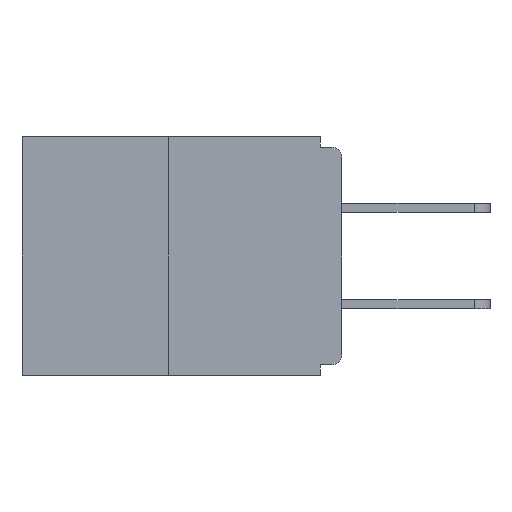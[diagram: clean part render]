
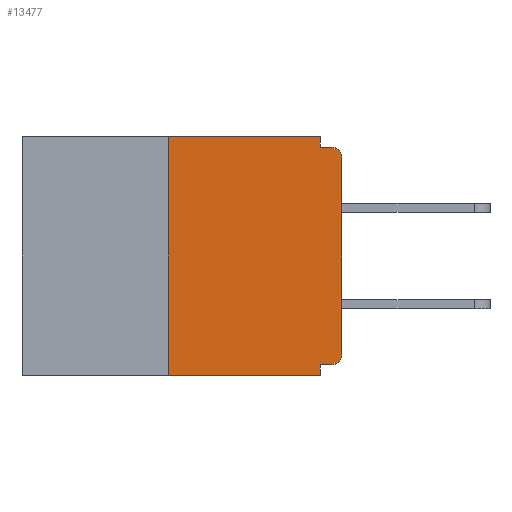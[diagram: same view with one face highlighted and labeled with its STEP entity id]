
A CAD part, left-side view. The second image highlights one B-rep face of the part: STEP entity #13477.
In plain terms, the highlighted planar face has unit normal (-1, 0, 0).
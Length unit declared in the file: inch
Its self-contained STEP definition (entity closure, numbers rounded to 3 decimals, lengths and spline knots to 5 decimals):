
#249 = CARTESIAN_POINT ( 'NONE',  ( 0., 0., -0.328 ) ) ;
#279 = DIRECTION ( 'NONE',  ( -1., 0., 0. ) ) ;
#351 = VERTEX_POINT ( 'NONE', #12477 ) ;
#446 = EDGE_CURVE ( 'NONE', #6713, #351, #14507, .T. ) ;
#727 = CARTESIAN_POINT ( 'NONE',  ( 0., 0.25, 0. ) ) ;
#910 = EDGE_CURVE ( 'NONE', #2890, #11654, #1604, .T. ) ;
#1026 = CARTESIAN_POINT ( 'NONE',  ( 0., 0.015, -0.015 ) ) ;
#1099 = ORIENTED_EDGE ( 'NONE', *, *, #910, .T. ) ;
#1271 = VERTEX_POINT ( 'NONE', #4079 ) ;
#1514 = DIRECTION ( 'NONE',  ( 0., 0., -1. ) ) ;
#1546 = AXIS2_PLACEMENT_3D ( 'NONE', #13833, #2771, #2620 ) ;
#1586 = CARTESIAN_POINT ( 'NONE',  ( 0., 0.031, -0.343 ) ) ;
#1604 = LINE ( 'NONE', #2665, #3016 ) ;
#1802 = DIRECTION ( 'NONE',  ( 0., 0., -1. ) ) ;
#1822 = DIRECTION ( 'NONE',  ( 0., 0., 1. ) ) ;
#2344 = VERTEX_POINT ( 'NONE', #13068 ) ;
#2375 = FACE_OUTER_BOUND ( 'NONE', #13878, .T. ) ;
#2427 = CIRCLE ( 'NONE', #1546, 0.015 ) ;
#2615 = DIRECTION ( 'NONE',  ( 0., -1., 0. ) ) ;
#2620 = DIRECTION ( 'NONE',  ( 0., 0., -1. ) ) ;
#2665 = CARTESIAN_POINT ( 'NONE',  ( 0., 0.46, -0.343 ) ) ;
#2771 = DIRECTION ( 'NONE',  ( -1., 0., 0. ) ) ;
#2811 = DIRECTION ( 'NONE',  ( 1., 0., 0. ) ) ;
#2890 = VERTEX_POINT ( 'NONE', #10307 ) ;
#2918 = VECTOR ( 'NONE', #1514, 39.37008 ) ;
#2968 = LINE ( 'NONE', #11982, #5103 ) ;
#3007 = AXIS2_PLACEMENT_3D ( 'NONE', #3463, #279, #7038 ) ;
#3016 = VECTOR ( 'NONE', #2615, 39.37008 ) ;
#3120 = LINE ( 'NONE', #3631, #12502 ) ;
#3336 = ORIENTED_EDGE ( 'NONE', *, *, #10011, .F. ) ;
#3463 = CARTESIAN_POINT ( 'NONE',  ( 0., 0.015, -0.03 ) ) ;
#3493 = EDGE_CURVE ( 'NONE', #2344, #8416, #2968, .T. ) ;
#3596 = CARTESIAN_POINT ( 'NONE',  ( 0., 0.031, -0.343 ) ) ;
#3631 = CARTESIAN_POINT ( 'NONE',  ( 0., 0.031, 0. ) ) ;
#4079 = CARTESIAN_POINT ( 'NONE',  ( 0., 0., -0.03 ) ) ;
#4272 = LINE ( 'NONE', #10530, #12057 ) ;
#4614 = DIRECTION ( 'NONE',  ( 0., 0., -1. ) ) ;
#4646 = VECTOR ( 'NONE', #7058, 39.37008 ) ;
#5100 = VERTEX_POINT ( 'NONE', #10645 ) ;
#5103 = VECTOR ( 'NONE', #10808, 39.37008 ) ;
#5326 = CARTESIAN_POINT ( 'NONE',  ( 0., 0.031, -0.015 ) ) ;
#5466 = AXIS2_PLACEMENT_3D ( 'NONE', #6154, #2811, #1802 ) ;
#5928 = ORIENTED_EDGE ( 'NONE', *, *, #12343, .F. ) ;
#5972 = EDGE_CURVE ( 'NONE', #1271, #14247, #12173, .T. ) ;
#6154 = CARTESIAN_POINT ( 'NONE',  ( 0., 0.46, 0. ) ) ;
#6713 = VERTEX_POINT ( 'NONE', #9523 ) ;
#6881 = DIRECTION ( 'NONE',  ( 0., 0., 1. ) ) ;
#6967 = ORIENTED_EDGE ( 'NONE', *, *, #11151, .T. ) ;
#7038 = DIRECTION ( 'NONE',  ( 0., 0., -1. ) ) ;
#7058 = DIRECTION ( 'NONE',  ( 0., 1., 0. ) ) ;
#8039 = ORIENTED_EDGE ( 'NONE', *, *, #5972, .T. ) ;
#8416 = VERTEX_POINT ( 'NONE', #11031 ) ;
#9334 = VECTOR ( 'NONE', #1822, 39.37008 ) ;
#9523 = CARTESIAN_POINT ( 'NONE',  ( 0., 0.015, -0.328 ) ) ;
#9799 = VECTOR ( 'NONE', #6881, 39.37008 ) ;
#10011 = EDGE_CURVE ( 'NONE', #13180, #14247, #4272, .T. ) ;
#10307 = CARTESIAN_POINT ( 'NONE',  ( 0., 0.25, -0.343 ) ) ;
#10530 = CARTESIAN_POINT ( 'NONE',  ( 0., 0., -0.015 ) ) ;
#10645 = CARTESIAN_POINT ( 'NONE',  ( 0., 0., -0.313 ) ) ;
#10792 = ORIENTED_EDGE ( 'NONE', *, *, #13257, .T. ) ;
#10808 = DIRECTION ( 'NONE',  ( 0., -1., 0. ) ) ;
#11031 = CARTESIAN_POINT ( 'NONE',  ( 0., 0.031, 0. ) ) ;
#11151 = EDGE_CURVE ( 'NONE', #6713, #5100, #2427, .T. ) ;
#11176 = ORIENTED_EDGE ( 'NONE', *, *, #3493, .F. ) ;
#11325 = EDGE_CURVE ( 'NONE', #2890, #2344, #11465, .T. ) ;
#11348 = ORIENTED_EDGE ( 'NONE', *, *, #11514, .F. ) ;
#11465 = LINE ( 'NONE', #727, #9334 ) ;
#11514 = EDGE_CURVE ( 'NONE', #8416, #13180, #3120, .T. ) ;
#11631 = ORIENTED_EDGE ( 'NONE', *, *, #11325, .F. ) ;
#11654 = VERTEX_POINT ( 'NONE', #1586 ) ;
#11982 = CARTESIAN_POINT ( 'NONE',  ( 0., 0.46, 0. ) ) ;
#12057 = VECTOR ( 'NONE', #12804, 39.37008 ) ;
#12173 = CIRCLE ( 'NONE', #3007, 0.015 ) ;
#12343 = EDGE_CURVE ( 'NONE', #351, #11654, #14213, .T. ) ;
#12477 = CARTESIAN_POINT ( 'NONE',  ( 0., 0.031, -0.328 ) ) ;
#12502 = VECTOR ( 'NONE', #4614, 39.37008 ) ;
#12804 = DIRECTION ( 'NONE',  ( 0., -1., 0. ) ) ;
#12818 = LINE ( 'NONE', #13577, #9799 ) ;
#13068 = CARTESIAN_POINT ( 'NONE',  ( 0., 0.25, 0. ) ) ;
#13131 = ORIENTED_EDGE ( 'NONE', *, *, #446, .F. ) ;
#13180 = VERTEX_POINT ( 'NONE', #5326 ) ;
#13257 = EDGE_CURVE ( 'NONE', #5100, #1271, #12818, .T. ) ;
#13477 = ADVANCED_FACE ( 'NONE', ( #2375 ), #14158, .F. ) ;
#13577 = CARTESIAN_POINT ( 'NONE',  ( 0., 0., 0. ) ) ;
#13833 = CARTESIAN_POINT ( 'NONE',  ( 0., 0.015, -0.313 ) ) ;
#13878 = EDGE_LOOP ( 'NONE', ( #11176, #11631, #1099, #5928, #13131, #6967, #10792, #8039, #3336, #11348 ) ) ;
#14158 = PLANE ( 'NONE',  #5466 ) ;
#14213 = LINE ( 'NONE', #3596, #2918 ) ;
#14247 = VERTEX_POINT ( 'NONE', #1026 ) ;
#14507 = LINE ( 'NONE', #249, #4646 ) ;
